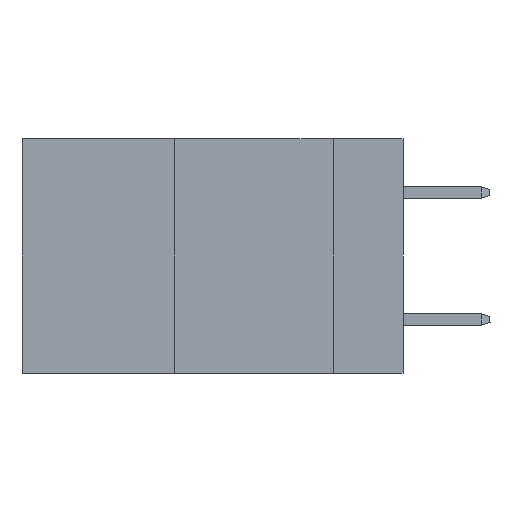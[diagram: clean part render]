
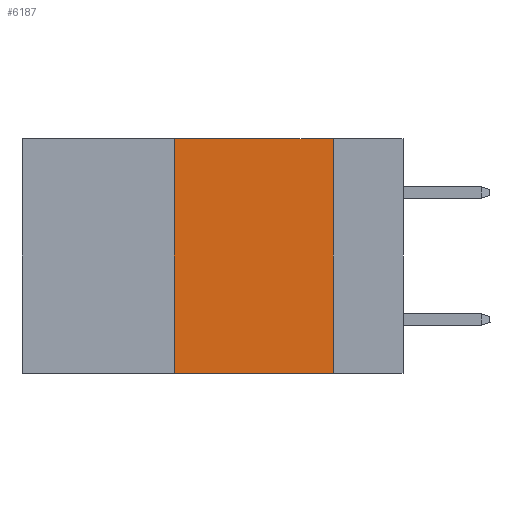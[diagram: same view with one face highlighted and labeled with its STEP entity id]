
A CAD part, left-side view. The second image highlights one B-rep face of the part: STEP entity #6187.
In plain terms, the highlighted planar face has unit normal (-1, 0, 0).
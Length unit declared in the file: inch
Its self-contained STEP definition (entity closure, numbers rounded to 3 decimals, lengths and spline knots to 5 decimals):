
#309 = LINE ( 'NONE', #15175, #494 ) ;
#494 = VECTOR ( 'NONE', #8714, 39.37008 ) ;
#559 = FACE_OUTER_BOUND ( 'NONE', #10423, .T. ) ;
#571 = LINE ( 'NONE', #8972, #26681 ) ;
#1057 = VERTEX_POINT ( 'NONE', #18898 ) ;
#2853 = LINE ( 'NONE', #26002, #15461 ) ;
#3364 = VERTEX_POINT ( 'NONE', #3806 ) ;
#3372 = ORIENTED_EDGE ( 'NONE', *, *, #5398, .F. ) ;
#3806 = CARTESIAN_POINT ( 'NONE',  ( 0., 0.11, -0.37 ) ) ;
#4844 = CARTESIAN_POINT ( 'NONE',  ( 0., 0.36, -0.37 ) ) ;
#5084 = LINE ( 'NONE', #17326, #7051 ) ;
#5398 = EDGE_CURVE ( 'NONE', #1057, #3364, #571, .T. ) ;
#6187 = ADVANCED_FACE ( 'NONE', ( #559 ), #17333, .F. ) ;
#7030 = DIRECTION ( 'NONE',  ( 1., 0., 0. ) ) ;
#7051 = VECTOR ( 'NONE', #11195, 39.37008 ) ;
#8714 = DIRECTION ( 'NONE',  ( 0., -1., 0. ) ) ;
#8926 = DIRECTION ( 'NONE',  ( 0., 0., 1. ) ) ;
#8972 = CARTESIAN_POINT ( 'NONE',  ( 0., 0.11, 0. ) ) ;
#9386 = DIRECTION ( 'NONE',  ( 0., 0., -1. ) ) ;
#9702 = EDGE_CURVE ( 'NONE', #26559, #1057, #5084, .T. ) ;
#10423 = EDGE_LOOP ( 'NONE', ( #3372, #23516, #19083, #23466 ) ) ;
#11195 = DIRECTION ( 'NONE',  ( 0., -1., 0. ) ) ;
#15175 = CARTESIAN_POINT ( 'NONE',  ( 0., 0.6, -0.37 ) ) ;
#15461 = VECTOR ( 'NONE', #8926, 39.37008 ) ;
#17299 = EDGE_CURVE ( 'NONE', #17358, #3364, #309, .T. ) ;
#17326 = CARTESIAN_POINT ( 'NONE',  ( 0., 0.6, 0. ) ) ;
#17333 = PLANE ( 'NONE',  #23668 ) ;
#17340 = CARTESIAN_POINT ( 'NONE',  ( 0., 0.36, 0. ) ) ;
#17358 = VERTEX_POINT ( 'NONE', #4844 ) ;
#17598 = CARTESIAN_POINT ( 'NONE',  ( 0., 0.6, 0. ) ) ;
#18113 = EDGE_CURVE ( 'NONE', #17358, #26559, #2853, .T. ) ;
#18898 = CARTESIAN_POINT ( 'NONE',  ( 0., 0.11, 0. ) ) ;
#19083 = ORIENTED_EDGE ( 'NONE', *, *, #18113, .F. ) ;
#19255 = DIRECTION ( 'NONE',  ( 0., 0., -1. ) ) ;
#23466 = ORIENTED_EDGE ( 'NONE', *, *, #17299, .T. ) ;
#23516 = ORIENTED_EDGE ( 'NONE', *, *, #9702, .F. ) ;
#23668 = AXIS2_PLACEMENT_3D ( 'NONE', #17598, #7030, #19255 ) ;
#26002 = CARTESIAN_POINT ( 'NONE',  ( 0., 0.36, 0. ) ) ;
#26559 = VERTEX_POINT ( 'NONE', #17340 ) ;
#26681 = VECTOR ( 'NONE', #9386, 39.37008 ) ;
